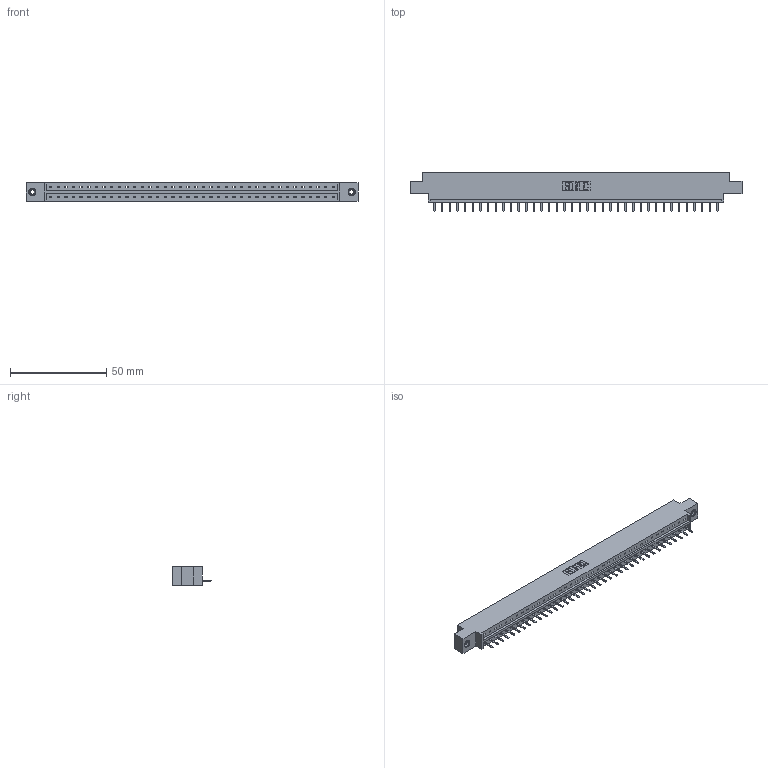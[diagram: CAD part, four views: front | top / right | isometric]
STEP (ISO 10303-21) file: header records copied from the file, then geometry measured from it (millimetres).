
FILE_DESCRIPTION (( 'STEP AP203' ), '1' );
FILE_NAME ('833-038-520-608.STEP', '2020-06-03T06:26:51', ( '' ), ( '' ), 'SwSTEP 2.0', 'SolidWorks 2020', '' );
FILE_SCHEMA (( 'CONFIG_CONTROL_DESIGN' ));
Length unit declared in the file: inch
Products named in the file (4): 833 Part_Offset - .156 Dia - TI; 345-292-001_345-293-120; 833-038-520-608; 345-250-001_345-250-003-102
Assembly tree (41 placements, depth 2):
  833-038-520-608
    833 Part_Offset - .156 Dia - TI
    345-292-001_345-293-120  x38
    345-250-001_345-250-003-102  x2
Bounding box: 172.11 x 20.02 x 9.4 mm (x, y, z)
Volume: 16941.1 mm3; surface area: 18144.3 mm2
Topology: 41 solids, 41 shells, 2534 faces, 7451 edges, 4858 vertices
Faces by surface type: plane 1778, cylinder 740, cone 12, torus 4
Entity records: 25180 total; most frequent: CARTESIAN_POINT 4339, ORIENTED_EDGE 4294, DIRECTION 3689, EDGE_CURVE 2147, LINE 1995, VECTOR 1995, VERTEX_POINT 1424, AXIS2_PLACEMENT_3D 847
